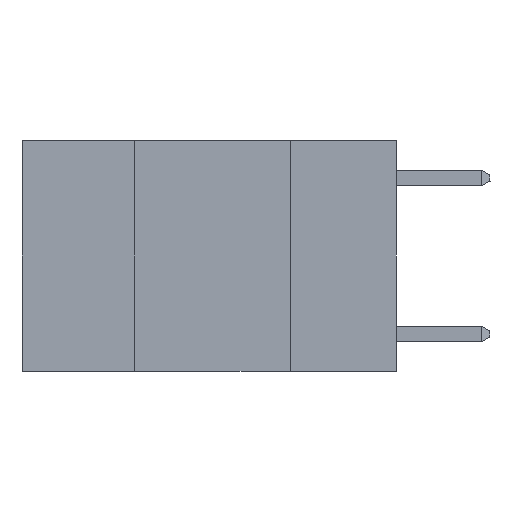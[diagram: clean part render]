
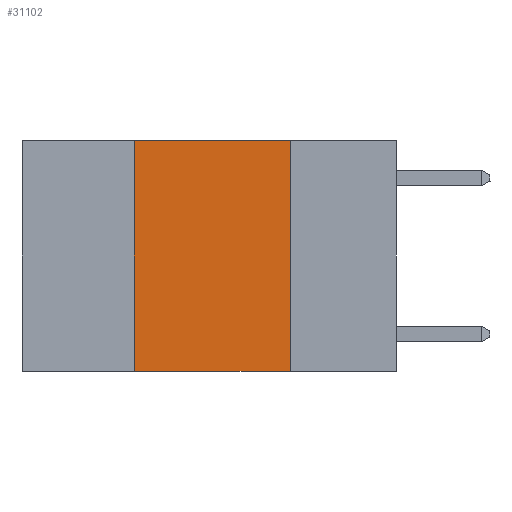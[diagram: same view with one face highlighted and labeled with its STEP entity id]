
A CAD part, left-side view. The second image highlights one B-rep face of the part: STEP entity #31102.
In plain terms, the highlighted planar face has unit normal (-1, 0, 0).
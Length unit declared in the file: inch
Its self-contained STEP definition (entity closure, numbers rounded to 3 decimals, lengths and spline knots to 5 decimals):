
#1047 = CARTESIAN_POINT ( 'NONE',  ( 0., 0.17, -0.37 ) ) ;
#1098 = CARTESIAN_POINT ( 'NONE',  ( 0., 0.42, 0. ) ) ;
#2588 = EDGE_CURVE ( 'NONE', #9788, #20250, #8682, .T. ) ;
#2723 = DIRECTION ( 'NONE',  ( 0., 0., -1. ) ) ;
#2801 = VERTEX_POINT ( 'NONE', #24987 ) ;
#3019 = CARTESIAN_POINT ( 'NONE',  ( 0., 0.6, -0.37 ) ) ;
#3176 = LINE ( 'NONE', #3019, #22094 ) ;
#3735 = EDGE_CURVE ( 'NONE', #2801, #5763, #3176, .T. ) ;
#4017 = DIRECTION ( 'NONE',  ( 0., 0., -1. ) ) ;
#5763 = VERTEX_POINT ( 'NONE', #1047 ) ;
#6722 = CARTESIAN_POINT ( 'NONE',  ( 0., 0.6, 0. ) ) ;
#7186 = CARTESIAN_POINT ( 'NONE',  ( 0., 0.42, 0. ) ) ;
#7623 = DIRECTION ( 'NONE',  ( 0., -1., 0. ) ) ;
#7712 = VECTOR ( 'NONE', #28021, 39.37008 ) ;
#8682 = LINE ( 'NONE', #18351, #7712 ) ;
#8947 = PLANE ( 'NONE',  #28773 ) ;
#9569 = LINE ( 'NONE', #7186, #25347 ) ;
#9788 = VERTEX_POINT ( 'NONE', #1098 ) ;
#11453 = VECTOR ( 'NONE', #2723, 39.37008 ) ;
#11469 = DIRECTION ( 'NONE',  ( 1., 0., 0. ) ) ;
#12415 = CARTESIAN_POINT ( 'NONE',  ( 0., 0.17, 0. ) ) ;
#12622 = ORIENTED_EDGE ( 'NONE', *, *, #14558, .F. ) ;
#14558 = EDGE_CURVE ( 'NONE', #20250, #5763, #20556, .T. ) ;
#15366 = ORIENTED_EDGE ( 'NONE', *, *, #2588, .F. ) ;
#16859 = DIRECTION ( 'NONE',  ( 0., 0., 1. ) ) ;
#17239 = CARTESIAN_POINT ( 'NONE',  ( 0., 0.17, 0. ) ) ;
#18228 = ORIENTED_EDGE ( 'NONE', *, *, #21083, .F. ) ;
#18351 = CARTESIAN_POINT ( 'NONE',  ( 0., 0.6, 0. ) ) ;
#20250 = VERTEX_POINT ( 'NONE', #17239 ) ;
#20556 = LINE ( 'NONE', #12415, #11453 ) ;
#20902 = EDGE_LOOP ( 'NONE', ( #12622, #15366, #18228, #27043 ) ) ;
#21083 = EDGE_CURVE ( 'NONE', #2801, #9788, #9569, .T. ) ;
#22094 = VECTOR ( 'NONE', #7623, 39.37008 ) ;
#23833 = FACE_OUTER_BOUND ( 'NONE', #20902, .T. ) ;
#24987 = CARTESIAN_POINT ( 'NONE',  ( 0., 0.42, -0.37 ) ) ;
#25347 = VECTOR ( 'NONE', #16859, 39.37008 ) ;
#27043 = ORIENTED_EDGE ( 'NONE', *, *, #3735, .T. ) ;
#28021 = DIRECTION ( 'NONE',  ( 0., -1., 0. ) ) ;
#28773 = AXIS2_PLACEMENT_3D ( 'NONE', #6722, #11469, #4017 ) ;
#31102 = ADVANCED_FACE ( 'NONE', ( #23833 ), #8947, .F. ) ;
